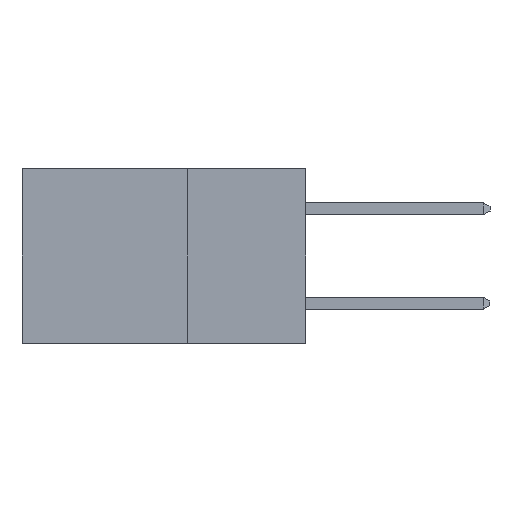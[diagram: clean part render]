
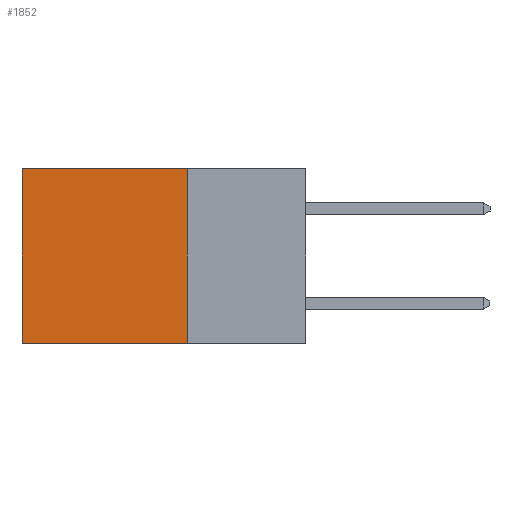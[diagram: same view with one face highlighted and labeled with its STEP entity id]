
A CAD part, left-side view. The second image highlights one B-rep face of the part: STEP entity #1852.
In plain terms, the highlighted planar face has unit normal (-1, 0, 0).
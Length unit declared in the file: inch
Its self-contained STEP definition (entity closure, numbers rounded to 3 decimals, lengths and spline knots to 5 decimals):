
#147 = EDGE_LOOP ( 'NONE', ( #4304, #6155, #247, #3723 ) ) ;
#247 = ORIENTED_EDGE ( 'NONE', *, *, #934, .F. ) ;
#562 = DIRECTION ( 'NONE',  ( 0., 0., -1. ) ) ;
#565 = FACE_OUTER_BOUND ( 'NONE', #147, .T. ) ;
#642 = CARTESIAN_POINT ( 'NONE',  ( 0.298, 0.6, 0. ) ) ;
#934 = EDGE_CURVE ( 'NONE', #2938, #3806, #2552, .T. ) ;
#967 = LINE ( 'NONE', #4513, #8952 ) ;
#1830 = EDGE_CURVE ( 'NONE', #3806, #8279, #5147, .T. ) ;
#1852 = ADVANCED_FACE ( 'NONE', ( #565 ), #7774, .F. ) ;
#2479 = CARTESIAN_POINT ( 'NONE',  ( 0.298, 0.25, 0. ) ) ;
#2532 = CARTESIAN_POINT ( 'NONE',  ( 0.298, 0.25, -0.37 ) ) ;
#2552 = LINE ( 'NONE', #5642, #4409 ) ;
#2938 = VERTEX_POINT ( 'NONE', #2479 ) ;
#3078 = CARTESIAN_POINT ( 'NONE',  ( 0.298, 0.6, 0. ) ) ;
#3478 = DIRECTION ( 'NONE',  ( 1., 0., 0. ) ) ;
#3699 = AXIS2_PLACEMENT_3D ( 'NONE', #6599, #3478, #8546 ) ;
#3723 = ORIENTED_EDGE ( 'NONE', *, *, #6448, .T. ) ;
#3806 = VERTEX_POINT ( 'NONE', #2532 ) ;
#4084 = DIRECTION ( 'NONE',  ( 0., 0., -1. ) ) ;
#4304 = ORIENTED_EDGE ( 'NONE', *, *, #6955, .T. ) ;
#4333 = VERTEX_POINT ( 'NONE', #3078 ) ;
#4409 = VECTOR ( 'NONE', #4084, 39.37008 ) ;
#4471 = DIRECTION ( 'NONE',  ( 0., 1., 0. ) ) ;
#4513 = CARTESIAN_POINT ( 'NONE',  ( 0.298, 0.25, 0. ) ) ;
#5147 = LINE ( 'NONE', #7673, #8838 ) ;
#5444 = DIRECTION ( 'NONE',  ( 0., 1., 0. ) ) ;
#5642 = CARTESIAN_POINT ( 'NONE',  ( 0.298, 0.25, 0. ) ) ;
#6155 = ORIENTED_EDGE ( 'NONE', *, *, #1830, .F. ) ;
#6448 = EDGE_CURVE ( 'NONE', #2938, #4333, #967, .T. ) ;
#6599 = CARTESIAN_POINT ( 'NONE',  ( 0.298, 0.25, 0. ) ) ;
#6847 = VECTOR ( 'NONE', #562, 39.37008 ) ;
#6955 = EDGE_CURVE ( 'NONE', #4333, #8279, #7072, .T. ) ;
#7072 = LINE ( 'NONE', #642, #6847 ) ;
#7673 = CARTESIAN_POINT ( 'NONE',  ( 0.298, 0.25, -0.37 ) ) ;
#7774 = PLANE ( 'NONE',  #3699 ) ;
#8279 = VERTEX_POINT ( 'NONE', #8609 ) ;
#8546 = DIRECTION ( 'NONE',  ( 0., 0., -1. ) ) ;
#8609 = CARTESIAN_POINT ( 'NONE',  ( 0.298, 0.6, -0.37 ) ) ;
#8838 = VECTOR ( 'NONE', #5444, 39.37008 ) ;
#8952 = VECTOR ( 'NONE', #4471, 39.37008 ) ;
